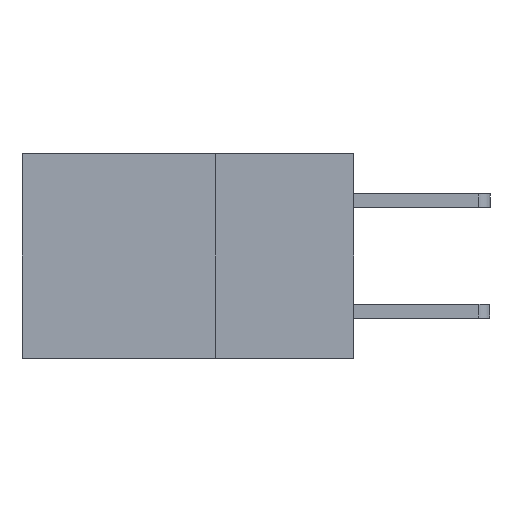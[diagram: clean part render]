
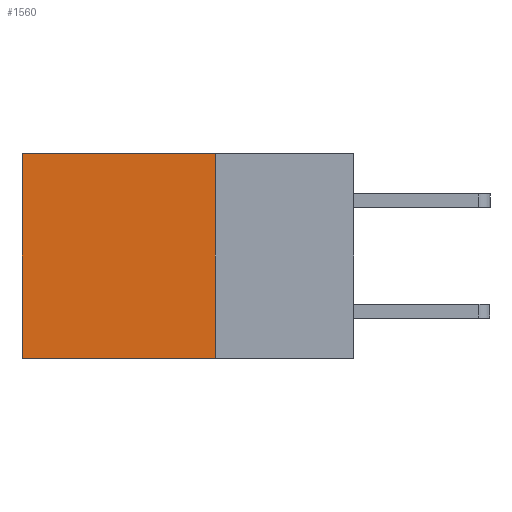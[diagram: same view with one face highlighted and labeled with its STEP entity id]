
A CAD part, left-side view. The second image highlights one B-rep face of the part: STEP entity #1560.
In plain terms, the highlighted planar face has unit normal (-1, 0, 0).
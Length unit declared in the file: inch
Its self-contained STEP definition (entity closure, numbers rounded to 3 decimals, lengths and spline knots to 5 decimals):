
#242 = CARTESIAN_POINT ( 'NONE',  ( 0.2875, 0.6, 0. ) ) ;
#524 = EDGE_CURVE ( 'NONE', #2520, #4341, #8540, .T. ) ;
#573 = EDGE_CURVE ( 'NONE', #8051, #9900, #4326, .T. ) ;
#741 = DIRECTION ( 'NONE',  ( 1., 0., 0. ) ) ;
#1456 = DIRECTION ( 'NONE',  ( 0., 1., 0. ) ) ;
#1501 = VECTOR ( 'NONE', #5952, 39.37008 ) ;
#1537 = CARTESIAN_POINT ( 'NONE',  ( 0.2875, 0.25, 0. ) ) ;
#1560 = ADVANCED_FACE ( 'NONE', ( #7004 ), #6142, .F. ) ;
#1860 = DIRECTION ( 'NONE',  ( 0., 1., 0. ) ) ;
#1915 = VECTOR ( 'NONE', #1860, 39.37008 ) ;
#1964 = VECTOR ( 'NONE', #1456, 39.37008 ) ;
#2520 = VERTEX_POINT ( 'NONE', #242 ) ;
#2913 = LINE ( 'NONE', #6448, #1915 ) ;
#3730 = AXIS2_PLACEMENT_3D ( 'NONE', #9670, #741, #4403 ) ;
#4326 = LINE ( 'NONE', #1537, #10940 ) ;
#4341 = VERTEX_POINT ( 'NONE', #9375 ) ;
#4403 = DIRECTION ( 'NONE',  ( 0., 0., -1. ) ) ;
#5952 = DIRECTION ( 'NONE',  ( 0., 0., -1. ) ) ;
#6142 = PLANE ( 'NONE',  #3730 ) ;
#6448 = CARTESIAN_POINT ( 'NONE',  ( 0.2875, 0.25, -0.37 ) ) ;
#6517 = ORIENTED_EDGE ( 'NONE', *, *, #524, .T. ) ;
#7004 = FACE_OUTER_BOUND ( 'NONE', #8418, .T. ) ;
#8051 = VERTEX_POINT ( 'NONE', #9951 ) ;
#8360 = ORIENTED_EDGE ( 'NONE', *, *, #8935, .F. ) ;
#8408 = LINE ( 'NONE', #10260, #1964 ) ;
#8418 = EDGE_LOOP ( 'NONE', ( #6517, #8360, #8976, #10180 ) ) ;
#8540 = LINE ( 'NONE', #9536, #1501 ) ;
#8592 = CARTESIAN_POINT ( 'NONE',  ( 0.2875, 0.25, -0.37 ) ) ;
#8935 = EDGE_CURVE ( 'NONE', #9900, #4341, #2913, .T. ) ;
#8976 = ORIENTED_EDGE ( 'NONE', *, *, #573, .F. ) ;
#9375 = CARTESIAN_POINT ( 'NONE',  ( 0.2875, 0.6, -0.37 ) ) ;
#9536 = CARTESIAN_POINT ( 'NONE',  ( 0.2875, 0.6, 0. ) ) ;
#9670 = CARTESIAN_POINT ( 'NONE',  ( 0.2875, 0.25, 0. ) ) ;
#9900 = VERTEX_POINT ( 'NONE', #8592 ) ;
#9951 = CARTESIAN_POINT ( 'NONE',  ( 0.2875, 0.25, 0. ) ) ;
#10180 = ORIENTED_EDGE ( 'NONE', *, *, #10321, .T. ) ;
#10260 = CARTESIAN_POINT ( 'NONE',  ( 0.2875, 0.25, 0. ) ) ;
#10321 = EDGE_CURVE ( 'NONE', #8051, #2520, #8408, .T. ) ;
#10940 = VECTOR ( 'NONE', #11147, 39.37008 ) ;
#11147 = DIRECTION ( 'NONE',  ( 0., 0., -1. ) ) ;
